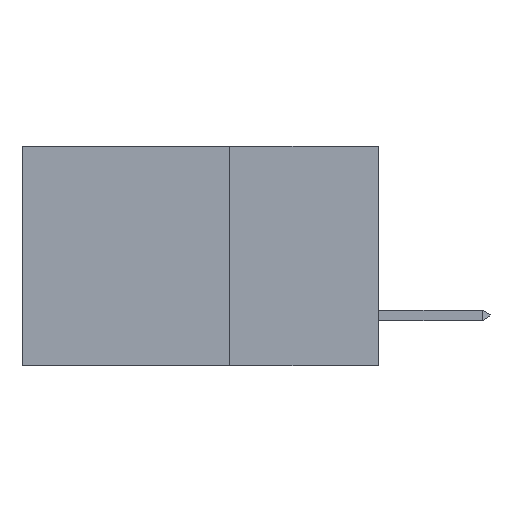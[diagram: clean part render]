
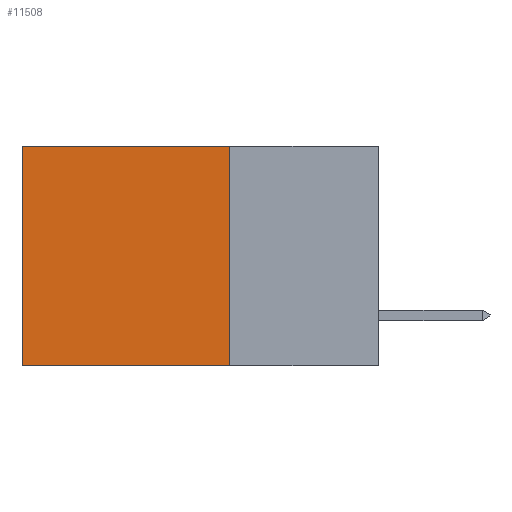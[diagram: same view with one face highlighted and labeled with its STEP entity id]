
A CAD part, left-side view. The second image highlights one B-rep face of the part: STEP entity #11508.
In plain terms, the highlighted planar face has unit normal (-1, 0, 0).
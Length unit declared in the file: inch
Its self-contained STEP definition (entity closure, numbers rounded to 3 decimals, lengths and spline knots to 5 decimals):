
#475 = PLANE ( 'NONE',  #21466 ) ;
#1386 = CARTESIAN_POINT ( 'NONE',  ( 0.298, 0.6, -0.37 ) ) ;
#2038 = EDGE_CURVE ( 'NONE', #11966, #6923, #2245, .T. ) ;
#2245 = LINE ( 'NONE', #6827, #16274 ) ;
#2392 = CARTESIAN_POINT ( 'NONE',  ( 0.298, 0.6, 0. ) ) ;
#3066 = EDGE_LOOP ( 'NONE', ( #10615, #13431, #16812, #3431 ) ) ;
#3431 = ORIENTED_EDGE ( 'NONE', *, *, #2038, .T. ) ;
#4725 = CARTESIAN_POINT ( 'NONE',  ( 0.298, 0.6, 0. ) ) ;
#5165 = CARTESIAN_POINT ( 'NONE',  ( 0.298, 0.25, 0. ) ) ;
#6316 = EDGE_CURVE ( 'NONE', #6923, #19543, #17175, .T. ) ;
#6827 = CARTESIAN_POINT ( 'NONE',  ( 0.298, 0.25, 0. ) ) ;
#6923 = VERTEX_POINT ( 'NONE', #2392 ) ;
#7593 = VECTOR ( 'NONE', #16331, 39.37008 ) ;
#8954 = DIRECTION ( 'NONE',  ( 1., 0., 0. ) ) ;
#10003 = DIRECTION ( 'NONE',  ( 0., 1., 0. ) ) ;
#10408 = EDGE_CURVE ( 'NONE', #11966, #20142, #19899, .T. ) ;
#10588 = DIRECTION ( 'NONE',  ( 0., 0., -1. ) ) ;
#10615 = ORIENTED_EDGE ( 'NONE', *, *, #6316, .T. ) ;
#11306 = CARTESIAN_POINT ( 'NONE',  ( 0.298, 0.25, -0.37 ) ) ;
#11508 = ADVANCED_FACE ( 'NONE', ( #17300 ), #475, .F. ) ;
#11966 = VERTEX_POINT ( 'NONE', #5165 ) ;
#12299 = EDGE_CURVE ( 'NONE', #20142, #19543, #20494, .T. ) ;
#13431 = ORIENTED_EDGE ( 'NONE', *, *, #12299, .F. ) ;
#13549 = DIRECTION ( 'NONE',  ( 0., 1., 0. ) ) ;
#15527 = VECTOR ( 'NONE', #20181, 39.37008 ) ;
#16274 = VECTOR ( 'NONE', #10003, 39.37008 ) ;
#16331 = DIRECTION ( 'NONE',  ( 0., 0., -1. ) ) ;
#16812 = ORIENTED_EDGE ( 'NONE', *, *, #10408, .F. ) ;
#16903 = VECTOR ( 'NONE', #13549, 39.37008 ) ;
#17042 = CARTESIAN_POINT ( 'NONE',  ( 0.298, 0.25, -0.37 ) ) ;
#17175 = LINE ( 'NONE', #4725, #7593 ) ;
#17300 = FACE_OUTER_BOUND ( 'NONE', #3066, .T. ) ;
#18678 = CARTESIAN_POINT ( 'NONE',  ( 0.298, 0.25, 0. ) ) ;
#18847 = CARTESIAN_POINT ( 'NONE',  ( 0.298, 0.25, 0. ) ) ;
#19543 = VERTEX_POINT ( 'NONE', #1386 ) ;
#19899 = LINE ( 'NONE', #18678, #15527 ) ;
#20142 = VERTEX_POINT ( 'NONE', #11306 ) ;
#20181 = DIRECTION ( 'NONE',  ( 0., 0., -1. ) ) ;
#20494 = LINE ( 'NONE', #17042, #16903 ) ;
#21466 = AXIS2_PLACEMENT_3D ( 'NONE', #18847, #8954, #10588 ) ;
